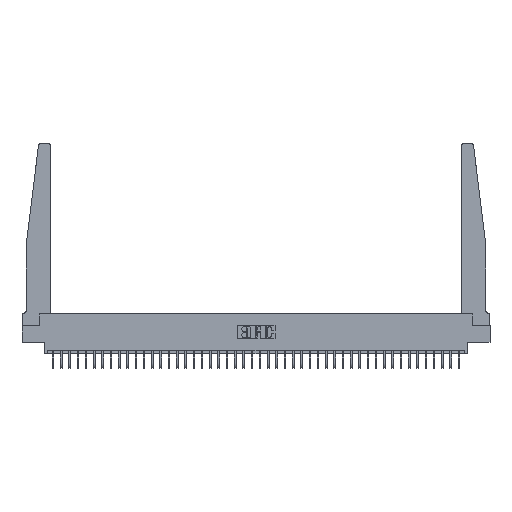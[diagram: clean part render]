
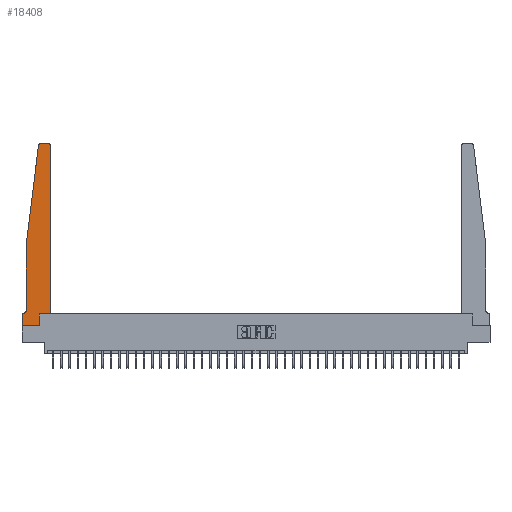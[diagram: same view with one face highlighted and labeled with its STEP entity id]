
A CAD part, top view. The second image highlights one B-rep face of the part: STEP entity #18408.
In plain terms, the highlighted planar face has unit normal (0, 0, 1).
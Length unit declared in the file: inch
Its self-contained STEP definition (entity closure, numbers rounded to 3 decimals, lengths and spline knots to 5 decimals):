
#369 = DIRECTION ( 'NONE',  ( 0., 0., 1. ) ) ;
#852 = VERTEX_POINT ( 'NONE', #31785 ) ;
#1794 = DIRECTION ( 'NONE',  ( -1., 0., 0. ) ) ;
#1977 = VERTEX_POINT ( 'NONE', #35643 ) ;
#2595 = ORIENTED_EDGE ( 'NONE', *, *, #21951, .T. ) ;
#2700 = ORIENTED_EDGE ( 'NONE', *, *, #14870, .T. ) ;
#3596 = CARTESIAN_POINT ( 'NONE',  ( 0.2605, 0., 0.37 ) ) ;
#4882 = ORIENTED_EDGE ( 'NONE', *, *, #24669, .T. ) ;
#5072 = VERTEX_POINT ( 'NONE', #34744 ) ;
#5076 = EDGE_CURVE ( 'NONE', #20603, #14434, #27541, .T. ) ;
#5629 = EDGE_CURVE ( 'NONE', #5072, #7208, #27948, .T. ) ;
#5643 = DIRECTION ( 'NONE',  ( -0.122, -0.992, 0. ) ) ;
#5651 = DIRECTION ( 'NONE',  ( 1., 0., 0. ) ) ;
#6260 = ORIENTED_EDGE ( 'NONE', *, *, #5076, .T. ) ;
#7208 = VERTEX_POINT ( 'NONE', #22889 ) ;
#7553 = VECTOR ( 'NONE', #20899, 39.37008 ) ;
#8239 = VECTOR ( 'NONE', #5643, 39.37008 ) ;
#8476 = LINE ( 'NONE', #22907, #36228 ) ;
#8884 = PLANE ( 'NONE',  #22146 ) ;
#8892 = LINE ( 'NONE', #15495, #29771 ) ;
#9440 = ORIENTED_EDGE ( 'NONE', *, *, #22621, .T. ) ;
#9961 = LINE ( 'NONE', #11201, #15500 ) ;
#10410 = ORIENTED_EDGE ( 'NONE', *, *, #32487, .T. ) ;
#10602 = AXIS2_PLACEMENT_3D ( 'NONE', #34615, #13509, #16884 ) ;
#10664 = ORIENTED_EDGE ( 'NONE', *, *, #28675, .T. ) ;
#10916 = CARTESIAN_POINT ( 'NONE',  ( 0.425, 2.72, 0.37 ) ) ;
#11201 = CARTESIAN_POINT ( 'NONE',  ( 0.065, 1.25, 0.37 ) ) ;
#11302 = ORIENTED_EDGE ( 'NONE', *, *, #13263, .T. ) ;
#11534 = VECTOR ( 'NONE', #24809, 39.37008 ) ;
#11883 = CARTESIAN_POINT ( 'NONE',  ( 0., 0.1875, 0.37 ) ) ;
#11884 = VERTEX_POINT ( 'NONE', #3596 ) ;
#12923 = FACE_OUTER_BOUND ( 'NONE', #26122, .T. ) ;
#13263 = EDGE_CURVE ( 'NONE', #25151, #17780, #30073, .T. ) ;
#13509 = DIRECTION ( 'NONE',  ( 0., 0., 1. ) ) ;
#14434 = VERTEX_POINT ( 'NONE', #32433 ) ;
#14870 = EDGE_CURVE ( 'NONE', #7208, #31913, #30843, .T. ) ;
#14886 = CARTESIAN_POINT ( 'NONE',  ( 0., 0., 0.37 ) ) ;
#14944 = CARTESIAN_POINT ( 'NONE',  ( 0.395, 2.72, 0.37 ) ) ;
#15495 = CARTESIAN_POINT ( 'NONE',  ( 0.2605, 0.18, 0.37 ) ) ;
#15500 = VECTOR ( 'NONE', #35212, 39.37008 ) ;
#15581 = VECTOR ( 'NONE', #20595, 39.37008 ) ;
#16673 = EDGE_CURVE ( 'NONE', #31913, #36671, #31622, .T. ) ;
#16884 = DIRECTION ( 'NONE',  ( 1., 0., 0. ) ) ;
#16917 = CARTESIAN_POINT ( 'NONE',  ( 0.015, 0.2375, 0.37 ) ) ;
#17015 = LINE ( 'NONE', #14886, #15581 ) ;
#17600 = VERTEX_POINT ( 'NONE', #36224 ) ;
#17780 = VERTEX_POINT ( 'NONE', #10916 ) ;
#18150 = CARTESIAN_POINT ( 'NONE',  ( 0., 0., 0.37 ) ) ;
#18190 = DIRECTION ( 'NONE',  ( 1., 0., 0. ) ) ;
#18408 = ADVANCED_FACE ( 'NONE', ( #12923 ), #8884, .T. ) ;
#18803 = CARTESIAN_POINT ( 'NONE',  ( 0.27653, 2.75, 0.37 ) ) ;
#18885 = CARTESIAN_POINT ( 'NONE',  ( 0.425, 0.18, 0.37 ) ) ;
#20595 = DIRECTION ( 'NONE',  ( 1., 0., 0. ) ) ;
#20603 = VERTEX_POINT ( 'NONE', #18803 ) ;
#20784 = CARTESIAN_POINT ( 'NONE',  ( 0., 0., 0.37 ) ) ;
#20899 = DIRECTION ( 'NONE',  ( 0., -1., 0. ) ) ;
#21038 = EDGE_CURVE ( 'NONE', #17780, #17600, #22975, .T. ) ;
#21187 = DIRECTION ( 'NONE',  ( 0., 1., 0. ) ) ;
#21425 = DIRECTION ( 'NONE',  ( 1., 0., 0. ) ) ;
#21951 = EDGE_CURVE ( 'NONE', #852, #5072, #9961, .T. ) ;
#22146 = AXIS2_PLACEMENT_3D ( 'NONE', #11883, #369, #21425 ) ;
#22621 = EDGE_CURVE ( 'NONE', #17600, #20603, #8476, .T. ) ;
#22756 = DIRECTION ( 'NONE',  ( -1., 0., 0. ) ) ;
#22889 = CARTESIAN_POINT ( 'NONE',  ( 0.015, 0.1875, 0.37 ) ) ;
#22907 = CARTESIAN_POINT ( 'NONE',  ( 0.25, 2.75, 0.37 ) ) ;
#22975 = CIRCLE ( 'NONE', #38055, 0.03 ) ;
#23950 = LINE ( 'NONE', #32402, #8239 ) ;
#24669 = EDGE_CURVE ( 'NONE', #36671, #11884, #17015, .T. ) ;
#24809 = DIRECTION ( 'NONE',  ( 0., 1., 0. ) ) ;
#25092 = ORIENTED_EDGE ( 'NONE', *, *, #32928, .T. ) ;
#25151 = VERTEX_POINT ( 'NONE', #33718 ) ;
#25435 = ORIENTED_EDGE ( 'NONE', *, *, #21038, .T. ) ;
#25864 = DIRECTION ( 'NONE',  ( -1., 0., 0. ) ) ;
#26122 = EDGE_LOOP ( 'NONE', ( #9440, #6260, #10664, #2595, #36077, #2700, #35111, #4882, #10410, #25092, #11302, #25435 ) ) ;
#27541 = CIRCLE ( 'NONE', #10602, 0.03 ) ;
#27948 = CIRCLE ( 'NONE', #30934, 0.05 ) ;
#28353 = CARTESIAN_POINT ( 'NONE',  ( 0.065, 0.1875, 0.37 ) ) ;
#28421 = DIRECTION ( 'NONE',  ( 0., 0., 1. ) ) ;
#28675 = EDGE_CURVE ( 'NONE', #14434, #852, #23950, .T. ) ;
#29771 = VECTOR ( 'NONE', #21187, 39.37008 ) ;
#30073 = LINE ( 'NONE', #18885, #11534 ) ;
#30323 = CARTESIAN_POINT ( 'NONE',  ( 0., 0.1875, 0.37 ) ) ;
#30843 = LINE ( 'NONE', #28353, #36361 ) ;
#30934 = AXIS2_PLACEMENT_3D ( 'NONE', #16917, #34249, #1794 ) ;
#31622 = LINE ( 'NONE', #20784, #7553 ) ;
#31785 = CARTESIAN_POINT ( 'NONE',  ( 0.065, 1.25, 0.37 ) ) ;
#31913 = VERTEX_POINT ( 'NONE', #30323 ) ;
#32402 = CARTESIAN_POINT ( 'NONE',  ( 0.065, 1.25, 0.37 ) ) ;
#32433 = CARTESIAN_POINT ( 'NONE',  ( 0.24675, 2.72367, 0.37 ) ) ;
#32487 = EDGE_CURVE ( 'NONE', #11884, #1977, #8892, .T. ) ;
#32928 = EDGE_CURVE ( 'NONE', #1977, #25151, #33398, .T. ) ;
#33398 = LINE ( 'NONE', #38229, #34342 ) ;
#33718 = CARTESIAN_POINT ( 'NONE',  ( 0.425, 0.18, 0.37 ) ) ;
#34249 = DIRECTION ( 'NONE',  ( 0., 0., -1. ) ) ;
#34342 = VECTOR ( 'NONE', #5651, 39.37008 ) ;
#34615 = CARTESIAN_POINT ( 'NONE',  ( 0.27653, 2.72, 0.37 ) ) ;
#34744 = CARTESIAN_POINT ( 'NONE',  ( 0.065, 0.2375, 0.37 ) ) ;
#35111 = ORIENTED_EDGE ( 'NONE', *, *, #16673, .T. ) ;
#35212 = DIRECTION ( 'NONE',  ( 0., -1., 0. ) ) ;
#35643 = CARTESIAN_POINT ( 'NONE',  ( 0.2605, 0.18, 0.37 ) ) ;
#36077 = ORIENTED_EDGE ( 'NONE', *, *, #5629, .T. ) ;
#36224 = CARTESIAN_POINT ( 'NONE',  ( 0.395, 2.75, 0.37 ) ) ;
#36228 = VECTOR ( 'NONE', #25864, 39.37008 ) ;
#36361 = VECTOR ( 'NONE', #22756, 39.37008 ) ;
#36671 = VERTEX_POINT ( 'NONE', #18150 ) ;
#38055 = AXIS2_PLACEMENT_3D ( 'NONE', #14944, #28421, #18190 ) ;
#38229 = CARTESIAN_POINT ( 'NONE',  ( 0.425, 0.18, 0.37 ) ) ;
